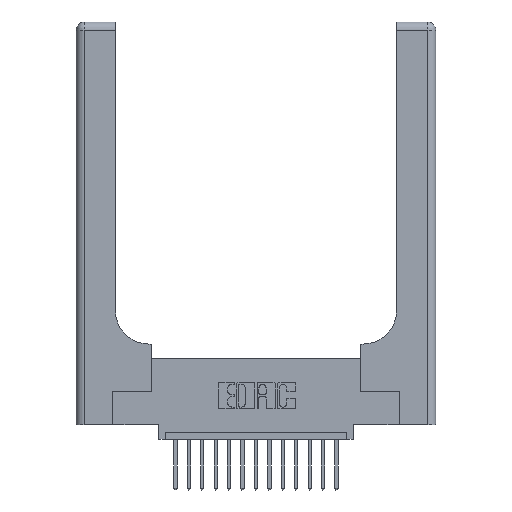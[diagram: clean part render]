
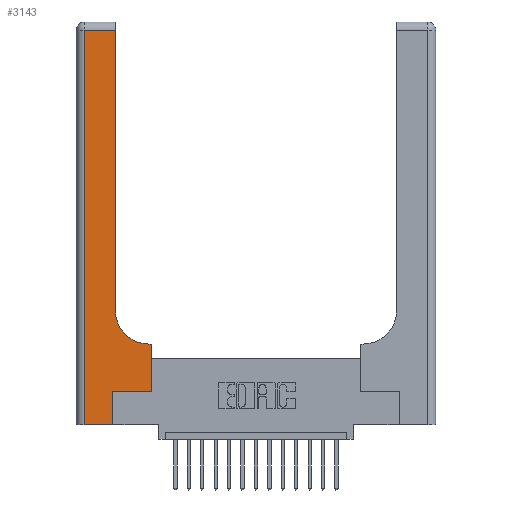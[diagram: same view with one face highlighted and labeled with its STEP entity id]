
A CAD part, top view. The second image highlights one B-rep face of the part: STEP entity #3143.
In plain terms, the highlighted planar face has unit normal (0, 0, 1).
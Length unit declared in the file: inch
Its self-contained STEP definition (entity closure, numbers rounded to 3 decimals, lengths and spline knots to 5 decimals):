
#37 = EDGE_CURVE ( 'NONE', #1741, #12632, #10164, .T. ) ;
#233 = CIRCLE ( 'NONE', #372, 0.25 ) ;
#372 = AXIS2_PLACEMENT_3D ( 'NONE', #4585, #7595, #431 ) ;
#388 = EDGE_CURVE ( 'NONE', #6546, #1741, #13587, .T. ) ;
#431 = DIRECTION ( 'NONE',  ( 1., 0., 0. ) ) ;
#475 = EDGE_CURVE ( 'NONE', #2743, #2985, #5960, .T. ) ;
#556 = DIRECTION ( 'NONE',  ( 0., 1., 0. ) ) ;
#744 = ORIENTED_EDGE ( 'NONE', *, *, #5805, .T. ) ;
#1029 = ORIENTED_EDGE ( 'NONE', *, *, #37, .T. ) ;
#1135 = FACE_OUTER_BOUND ( 'NONE', #2608, .T. ) ;
#1149 = EDGE_CURVE ( 'NONE', #10729, #3394, #1433, .T. ) ;
#1433 = LINE ( 'NONE', #12643, #9654 ) ;
#1526 = VERTEX_POINT ( 'NONE', #11683 ) ;
#1741 = VERTEX_POINT ( 'NONE', #8624 ) ;
#1857 = EDGE_CURVE ( 'NONE', #3394, #2743, #5544, .T. ) ;
#2054 = EDGE_CURVE ( 'NONE', #12632, #1526, #233, .T. ) ;
#2608 = EDGE_LOOP ( 'NONE', ( #18620, #744, #4573, #3888, #9910, #5694, #4435, #1029, #15727 ) ) ;
#2743 = VERTEX_POINT ( 'NONE', #7700 ) ;
#2973 = CARTESIAN_POINT ( 'NONE',  ( 0., 2.94, 0.37 ) ) ;
#2985 = VERTEX_POINT ( 'NONE', #15618 ) ;
#3143 = ADVANCED_FACE ( 'NONE', ( #1135 ), #14961, .F. ) ;
#3242 = DIRECTION ( 'NONE',  ( -1., 0., 0. ) ) ;
#3372 = DIRECTION ( 'NONE',  ( 0., 0., -1. ) ) ;
#3394 = VERTEX_POINT ( 'NONE', #13270 ) ;
#3497 = VECTOR ( 'NONE', #5402, 39.37008 ) ;
#3750 = VECTOR ( 'NONE', #17813, 39.37008 ) ;
#3888 = ORIENTED_EDGE ( 'NONE', *, *, #1857, .T. ) ;
#3948 = DIRECTION ( 'NONE',  ( 1., 0., 0. ) ) ;
#4173 = LINE ( 'NONE', #9177, #11522 ) ;
#4435 = ORIENTED_EDGE ( 'NONE', *, *, #388, .T. ) ;
#4573 = ORIENTED_EDGE ( 'NONE', *, *, #1149, .T. ) ;
#4585 = CARTESIAN_POINT ( 'NONE',  ( 0.5415, 0.85, 0.37 ) ) ;
#5402 = DIRECTION ( 'NONE',  ( 0., 1., 0. ) ) ;
#5452 = CARTESIAN_POINT ( 'NONE',  ( 0.2915, 2.94, 0.37 ) ) ;
#5487 = CARTESIAN_POINT ( 'NONE',  ( 0., 3., 0.37 ) ) ;
#5544 = LINE ( 'NONE', #12166, #15440 ) ;
#5554 = CARTESIAN_POINT ( 'NONE',  ( 0.06, 2.94, 0.37 ) ) ;
#5694 = ORIENTED_EDGE ( 'NONE', *, *, #14739, .T. ) ;
#5805 = EDGE_CURVE ( 'NONE', #10327, #10729, #15467, .T. ) ;
#5960 = LINE ( 'NONE', #9891, #16573 ) ;
#6164 = CARTESIAN_POINT ( 'NONE',  ( 0.269, 0.25, 0.37 ) ) ;
#6546 = VERTEX_POINT ( 'NONE', #16897 ) ;
#7595 = DIRECTION ( 'NONE',  ( 0., 0., -1. ) ) ;
#7700 = CARTESIAN_POINT ( 'NONE',  ( 0.269, 0., 0.37 ) ) ;
#8551 = CARTESIAN_POINT ( 'NONE',  ( 0.5585, 0.25, 0.37 ) ) ;
#8567 = VECTOR ( 'NONE', #10830, 39.37008 ) ;
#8624 = CARTESIAN_POINT ( 'NONE',  ( 0.5585, 0.6, 0.37 ) ) ;
#9177 = CARTESIAN_POINT ( 'NONE',  ( 0.2915, 3., 0.37 ) ) ;
#9654 = VECTOR ( 'NONE', #17004, 39.37008 ) ;
#9891 = CARTESIAN_POINT ( 'NONE',  ( 0.269, 0., 0.37 ) ) ;
#9910 = ORIENTED_EDGE ( 'NONE', *, *, #475, .T. ) ;
#10164 = LINE ( 'NONE', #13216, #12000 ) ;
#10327 = VERTEX_POINT ( 'NONE', #5452 ) ;
#10729 = VERTEX_POINT ( 'NONE', #5554 ) ;
#10830 = DIRECTION ( 'NONE',  ( 1., 0., 0. ) ) ;
#11088 = AXIS2_PLACEMENT_3D ( 'NONE', #5487, #3372, #3242 ) ;
#11522 = VECTOR ( 'NONE', #556, 39.37008 ) ;
#11670 = DIRECTION ( 'NONE',  ( -1., 0., 0. ) ) ;
#11675 = CARTESIAN_POINT ( 'NONE',  ( 0.5415, 0.6, 0.37 ) ) ;
#11683 = CARTESIAN_POINT ( 'NONE',  ( 0.2915, 0.85, 0.37 ) ) ;
#12000 = VECTOR ( 'NONE', #11670, 39.37008 ) ;
#12166 = CARTESIAN_POINT ( 'NONE',  ( 0., 0., 0.37 ) ) ;
#12632 = VERTEX_POINT ( 'NONE', #11675 ) ;
#12643 = CARTESIAN_POINT ( 'NONE',  ( 0.06, 3., 0.37 ) ) ;
#13216 = CARTESIAN_POINT ( 'NONE',  ( 0.2915, 0.6, 0.37 ) ) ;
#13270 = CARTESIAN_POINT ( 'NONE',  ( 0.06, 0., 0.37 ) ) ;
#13587 = LINE ( 'NONE', #8551, #3497 ) ;
#14739 = EDGE_CURVE ( 'NONE', #2985, #6546, #16389, .T. ) ;
#14961 = PLANE ( 'NONE',  #11088 ) ;
#15440 = VECTOR ( 'NONE', #3948, 39.37008 ) ;
#15467 = LINE ( 'NONE', #2973, #3750 ) ;
#15618 = CARTESIAN_POINT ( 'NONE',  ( 0.269, 0.25, 0.37 ) ) ;
#15727 = ORIENTED_EDGE ( 'NONE', *, *, #2054, .T. ) ;
#16389 = LINE ( 'NONE', #6164, #8567 ) ;
#16573 = VECTOR ( 'NONE', #17390, 39.37008 ) ;
#16897 = CARTESIAN_POINT ( 'NONE',  ( 0.5585, 0.25, 0.37 ) ) ;
#17004 = DIRECTION ( 'NONE',  ( 0., -1., 0. ) ) ;
#17390 = DIRECTION ( 'NONE',  ( 0., 1., 0. ) ) ;
#17813 = DIRECTION ( 'NONE',  ( -1., 0., 0. ) ) ;
#18446 = EDGE_CURVE ( 'NONE', #1526, #10327, #4173, .T. ) ;
#18620 = ORIENTED_EDGE ( 'NONE', *, *, #18446, .T. ) ;
